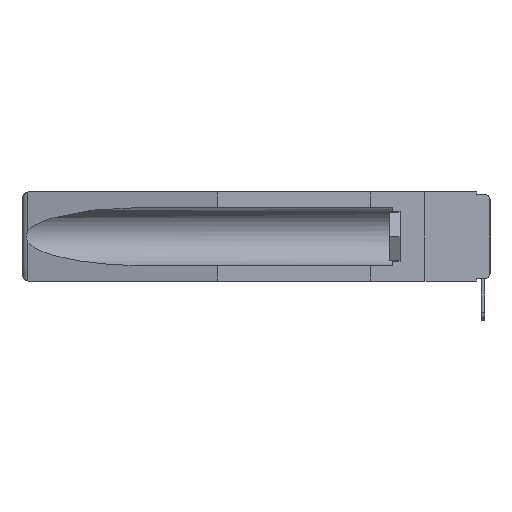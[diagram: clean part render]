
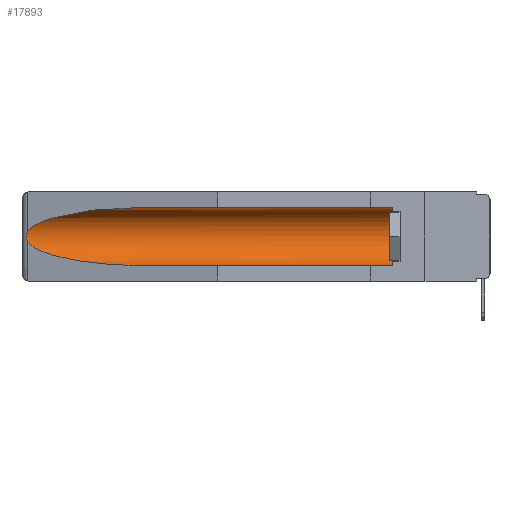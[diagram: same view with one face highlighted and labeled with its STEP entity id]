
A CAD part, left-side view. The second image highlights one B-rep face of the part: STEP entity #17893.
In plain terms, the highlighted cylindrical face has radius 2.857 mm (diameter 5.715 mm), a partial arc.
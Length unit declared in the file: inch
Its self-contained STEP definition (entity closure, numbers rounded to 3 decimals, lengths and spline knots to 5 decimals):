
#1149 = CARTESIAN_POINT ( 'NONE',  ( 0.26655, 1.53094, -0.18657 ) ) ;
#1157 = ORIENTED_EDGE ( 'NONE', *, *, #7341, .T. ) ;
#1217 = CARTESIAN_POINT ( 'NONE',  ( 0.155, 0.126, -0.1715 ) ) ;
#1265 = CARTESIAN_POINT ( 'NONE',  ( 0.2673, 1.53269, -0.17917 ) ) ;
#2598 = VECTOR ( 'NONE', #5302, 39.37008 ) ;
#3012 = CYLINDRICAL_SURFACE ( 'NONE', #6126, 0.1125 ) ;
#3045 = EDGE_CURVE ( 'NONE', #16543, #21215, #14766, .T. ) ;
#3982 = CARTESIAN_POINT ( 'NONE',  ( 0.26537, 1.52718, -0.19328 ) ) ;
#4910 = CARTESIAN_POINT ( 'NONE',  ( 0.26597, 1.5296, -0.19026 ) ) ;
#5302 = DIRECTION ( 'NONE',  ( 0., 1., 0. ) ) ;
#5340 = CARTESIAN_POINT ( 'NONE',  ( 0.155, 0.126, -0.284 ) ) ;
#6126 = AXIS2_PLACEMENT_3D ( 'NONE', #17497, #6767, #10418 ) ;
#6557 = CARTESIAN_POINT ( 'NONE',  ( 0.26537, 1.52718, -0.19328 ) ) ;
#6564 = VERTEX_POINT ( 'NONE', #13637 ) ;
#6767 = DIRECTION ( 'NONE',  ( 0., 1., 0. ) ) ;
#6796 = CARTESIAN_POINT ( 'NONE',  ( 0.155, 1.07973, -0.284 ) ) ;
#7223 = CARTESIAN_POINT ( 'NONE',  ( 0.26537, 1.52718, -0.14972 ) ) ;
#7341 = EDGE_CURVE ( 'NONE', #6564, #16543, #21402, .T. ) ;
#8029 = CARTESIAN_POINT ( 'NONE',  ( 0.26537, 1.52718, -0.14972 ) ) ;
#8265 = DIRECTION ( 'NONE',  ( 0., 0., 1. ) ) ;
#8874 = ORIENTED_EDGE ( 'NONE', *, *, #11089, .T. ) ;
#9298 = CARTESIAN_POINT ( 'NONE',  ( 0.26537, 1.52718, -0.14972 ) ) ;
#9851 = ORIENTED_EDGE ( 'NONE', *, *, #16444, .T. ) ;
#10418 = DIRECTION ( 'NONE',  ( 0., 0., 1. ) ) ;
#10751 = CARTESIAN_POINT ( 'NONE',  ( 0.21114, 1.30732, -0.059 ) ) ;
#10949 = EDGE_CURVE ( 'NONE', #16222, #14641, #17918, .T. ) ;
#11089 = EDGE_CURVE ( 'NONE', #21215, #18905, #17378, .T. ) ;
#12198 = CARTESIAN_POINT ( 'NONE',  ( 0.25451, 1.48313, -0.24835 ) ) ;
#12289 = CARTESIAN_POINT ( 'NONE',  ( 0.155, 1.07973, -0.059 ) ) ;
#13637 = CARTESIAN_POINT ( 'NONE',  ( 0.155, 0.126, -0.059 ) ) ;
#13652 = CIRCLE ( 'NONE', #20027, 0.1125 ) ;
#13962 = ORIENTED_EDGE ( 'NONE', *, *, #10949, .F. ) ;
#14128 = DIRECTION ( 'NONE',  ( 0., 1., 0. ) ) ;
#14641 = VERTEX_POINT ( 'NONE', #15729 ) ;
#14713 = CARTESIAN_POINT ( 'NONE',  ( 0.26654, 1.53092, -0.15636 ) ) ;
#14766 =( BOUNDED_CURVE ( )  B_SPLINE_CURVE ( 3, ( #12289, #10751, #19388, #7223 ),
 .UNSPECIFIED., .F., .F. ) 
 B_SPLINE_CURVE_WITH_KNOTS ( ( 4, 4 ),
 ( 4.71239, 6.08839 ),
 .UNSPECIFIED. ) 
 CURVE ( )  GEOMETRIC_REPRESENTATION_ITEM ( )  RATIONAL_B_SPLINE_CURVE ( ( 1., 0.848, 0.848, 1. ) ) 
 REPRESENTATION_ITEM ( '' )  );
#15336 = DIRECTION ( 'NONE',  ( 0., -1., 0. ) ) ;
#15599 = FACE_OUTER_BOUND ( 'NONE', #22307, .T. ) ;
#15729 = CARTESIAN_POINT ( 'NONE',  ( 0.155, 1.07973, -0.284 ) ) ;
#16222 = VERTEX_POINT ( 'NONE', #5340 ) ;
#16225 = CARTESIAN_POINT ( 'NONE',  ( 0.155, -0.30754, -0.059 ) ) ;
#16444 = EDGE_CURVE ( 'NONE', #16222, #6564, #13652, .T. ) ;
#16468 = CARTESIAN_POINT ( 'NONE',  ( 0.26597, 1.52961, -0.15275 ) ) ;
#16543 = VERTEX_POINT ( 'NONE', #22537 ) ;
#17181 =( BOUNDED_CURVE ( )  B_SPLINE_CURVE ( 3, ( #17519, #12198, #19406, #6796 ),
 .UNSPECIFIED., .F., .F. ) 
 B_SPLINE_CURVE_WITH_KNOTS ( ( 4, 4 ),
 ( 0.1948, 1.5708 ),
 .UNSPECIFIED. ) 
 CURVE ( )  GEOMETRIC_REPRESENTATION_ITEM ( )  RATIONAL_B_SPLINE_CURVE ( ( 1., 0.848, 0.848, 1. ) ) 
 REPRESENTATION_ITEM ( '' )  );
#17378 = B_SPLINE_CURVE_WITH_KNOTS ( 'NONE', 3,
 ( #9298, #16468, #14713, #21901, #19510, #21265, #1265, #1149, #4910, #6557 ),
 .UNSPECIFIED., .F., .F.,
 ( 4, 2, 2, 2, 4 ),
 ( 0., 0.00029, 0.00058, 0.00087, 0.00117 ),
 .UNSPECIFIED. ) ;
#17485 = EDGE_CURVE ( 'NONE', #18905, #14641, #17181, .T. ) ;
#17497 = CARTESIAN_POINT ( 'NONE',  ( 0.155, -0.30754, -0.1715 ) ) ;
#17519 = CARTESIAN_POINT ( 'NONE',  ( 0.26537, 1.52718, -0.19328 ) ) ;
#17893 = ADVANCED_FACE ( 'NONE', ( #15599 ), #3012, .F. ) ;
#17918 = LINE ( 'NONE', #21423, #2598 ) ;
#18686 = VECTOR ( 'NONE', #14128, 39.37008 ) ;
#18905 = VERTEX_POINT ( 'NONE', #3982 ) ;
#19388 = CARTESIAN_POINT ( 'NONE',  ( 0.25451, 1.48313, -0.09465 ) ) ;
#19406 = CARTESIAN_POINT ( 'NONE',  ( 0.21114, 1.30732, -0.284 ) ) ;
#19510 = CARTESIAN_POINT ( 'NONE',  ( 0.2675, 1.53308, -0.16763 ) ) ;
#19682 = ORIENTED_EDGE ( 'NONE', *, *, #3045, .T. ) ;
#20027 = AXIS2_PLACEMENT_3D ( 'NONE', #1217, #15336, #8265 ) ;
#21215 = VERTEX_POINT ( 'NONE', #8029 ) ;
#21265 = CARTESIAN_POINT ( 'NONE',  ( 0.2675, 1.53308, -0.17534 ) ) ;
#21402 = LINE ( 'NONE', #16225, #18686 ) ;
#21423 = CARTESIAN_POINT ( 'NONE',  ( 0.155, -0.30754, -0.284 ) ) ;
#21901 = CARTESIAN_POINT ( 'NONE',  ( 0.2673, 1.5327, -0.16383 ) ) ;
#22307 = EDGE_LOOP ( 'NONE', ( #19682, #8874, #22458, #13962, #9851, #1157 ) ) ;
#22458 = ORIENTED_EDGE ( 'NONE', *, *, #17485, .T. ) ;
#22537 = CARTESIAN_POINT ( 'NONE',  ( 0.155, 1.07973, -0.059 ) ) ;
